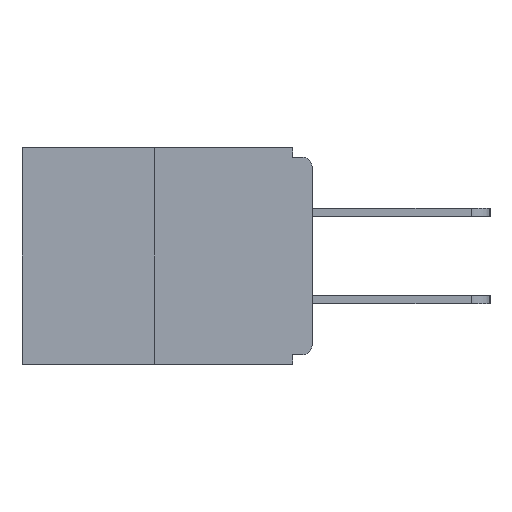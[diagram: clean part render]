
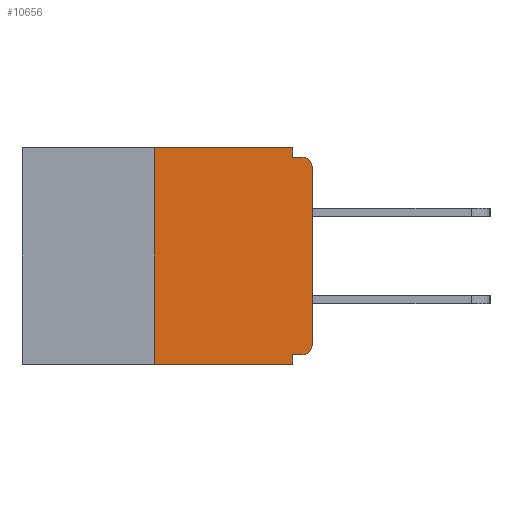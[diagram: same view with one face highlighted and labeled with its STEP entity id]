
A CAD part, left-side view. The second image highlights one B-rep face of the part: STEP entity #10656.
In plain terms, the highlighted planar face has unit normal (-1, 0, 0).
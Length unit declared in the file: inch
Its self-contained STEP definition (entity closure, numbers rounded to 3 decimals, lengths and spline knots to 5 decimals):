
#269 = VERTEX_POINT ( 'NONE', #14708 ) ;
#321 = LINE ( 'NONE', #11312, #3294 ) ;
#499 = VECTOR ( 'NONE', #761, 39.37008 ) ;
#652 = LINE ( 'NONE', #10535, #11108 ) ;
#732 = DIRECTION ( 'NONE',  ( 0., -1., 0. ) ) ;
#761 = DIRECTION ( 'NONE',  ( 0., 0., -1. ) ) ;
#832 = EDGE_CURVE ( 'NONE', #15999, #13995, #10374, .T. ) ;
#1209 = PLANE ( 'NONE',  #2395 ) ;
#1759 = VECTOR ( 'NONE', #14114, 39.37008 ) ;
#1936 = CARTESIAN_POINT ( 'NONE',  ( 0., 0., -0.015 ) ) ;
#2369 = EDGE_CURVE ( 'NONE', #269, #11917, #4774, .T. ) ;
#2395 = AXIS2_PLACEMENT_3D ( 'NONE', #10251, #11724, #10122 ) ;
#2478 = ORIENTED_EDGE ( 'NONE', *, *, #14129, .T. ) ;
#3040 = DIRECTION ( 'NONE',  ( -1., 0., 0. ) ) ;
#3227 = EDGE_LOOP ( 'NONE', ( #15905, #7117, #5791, #7458, #13691, #15611, #5646, #2478, #8967, #14660 ) ) ;
#3228 = AXIS2_PLACEMENT_3D ( 'NONE', #17382, #3040, #4282 ) ;
#3294 = VECTOR ( 'NONE', #17302, 39.37008 ) ;
#3340 = DIRECTION ( 'NONE',  ( 0., 0., 1. ) ) ;
#3433 = LINE ( 'NONE', #5644, #18622 ) ;
#4282 = DIRECTION ( 'NONE',  ( 0., 0., -1. ) ) ;
#4419 = VERTEX_POINT ( 'NONE', #15885 ) ;
#4670 = VECTOR ( 'NONE', #732, 39.37008 ) ;
#4696 = LINE ( 'NONE', #17206, #7650 ) ;
#4774 = LINE ( 'NONE', #10474, #15256 ) ;
#4870 = DIRECTION ( 'NONE',  ( 0., 0., -1. ) ) ;
#5045 = CARTESIAN_POINT ( 'NONE',  ( 0., 0.031, 0. ) ) ;
#5542 = CARTESIAN_POINT ( 'NONE',  ( 0., 0.031, 0. ) ) ;
#5644 = CARTESIAN_POINT ( 'NONE',  ( 0., 0.46, 0. ) ) ;
#5646 = ORIENTED_EDGE ( 'NONE', *, *, #15625, .T. ) ;
#5791 = ORIENTED_EDGE ( 'NONE', *, *, #15986, .T. ) ;
#6509 = LINE ( 'NONE', #12842, #1759 ) ;
#7117 = ORIENTED_EDGE ( 'NONE', *, *, #12773, .F. ) ;
#7458 = ORIENTED_EDGE ( 'NONE', *, *, #2369, .F. ) ;
#7491 = CIRCLE ( 'NONE', #3228, 0.015 ) ;
#7543 = DIRECTION ( 'NONE',  ( -1., 0., 0. ) ) ;
#7650 = VECTOR ( 'NONE', #12997, 39.37008 ) ;
#8511 = CARTESIAN_POINT ( 'NONE',  ( 0., 0.031, -0.015 ) ) ;
#8608 = VERTEX_POINT ( 'NONE', #10536 ) ;
#8967 = ORIENTED_EDGE ( 'NONE', *, *, #832, .F. ) ;
#9833 = EDGE_CURVE ( 'NONE', #15974, #269, #321, .T. ) ;
#10122 = DIRECTION ( 'NONE',  ( 0., 0., -1. ) ) ;
#10251 = CARTESIAN_POINT ( 'NONE',  ( 0., 0.46, 0. ) ) ;
#10374 = LINE ( 'NONE', #1936, #4670 ) ;
#10377 = CARTESIAN_POINT ( 'NONE',  ( 0., 0.015, -0.015 ) ) ;
#10474 = CARTESIAN_POINT ( 'NONE',  ( 0., 0.031, -0.343 ) ) ;
#10514 = CIRCLE ( 'NONE', #13297, 0.015 ) ;
#10535 = CARTESIAN_POINT ( 'NONE',  ( 0., 0.25, 0. ) ) ;
#10536 = CARTESIAN_POINT ( 'NONE',  ( 0., 0.25, -0.343 ) ) ;
#10656 = ADVANCED_FACE ( 'NONE', ( #10712 ), #1209, .F. ) ;
#10712 = FACE_OUTER_BOUND ( 'NONE', #3227, .T. ) ;
#10724 = CARTESIAN_POINT ( 'NONE',  ( 0., 0.015, -0.313 ) ) ;
#10970 = EDGE_CURVE ( 'NONE', #12462, #15999, #11608, .T. ) ;
#11108 = VECTOR ( 'NONE', #3340, 39.37008 ) ;
#11312 = CARTESIAN_POINT ( 'NONE',  ( 0., 0., -0.328 ) ) ;
#11608 = LINE ( 'NONE', #5045, #499 ) ;
#11687 = CARTESIAN_POINT ( 'NONE',  ( 0., 0.25, 0. ) ) ;
#11724 = DIRECTION ( 'NONE',  ( 1., 0., 0. ) ) ;
#11917 = VERTEX_POINT ( 'NONE', #18630 ) ;
#12240 = CARTESIAN_POINT ( 'NONE',  ( 0., 0.015, -0.328 ) ) ;
#12462 = VERTEX_POINT ( 'NONE', #5542 ) ;
#12553 = VERTEX_POINT ( 'NONE', #11687 ) ;
#12773 = EDGE_CURVE ( 'NONE', #8608, #12553, #652, .T. ) ;
#12842 = CARTESIAN_POINT ( 'NONE',  ( 0., 0.46, -0.343 ) ) ;
#12997 = DIRECTION ( 'NONE',  ( 0., 0., 1. ) ) ;
#13297 = AXIS2_PLACEMENT_3D ( 'NONE', #10724, #7543, #4870 ) ;
#13691 = ORIENTED_EDGE ( 'NONE', *, *, #9833, .F. ) ;
#13995 = VERTEX_POINT ( 'NONE', #10377 ) ;
#14114 = DIRECTION ( 'NONE',  ( 0., -1., 0. ) ) ;
#14129 = EDGE_CURVE ( 'NONE', #18629, #13995, #7491, .T. ) ;
#14409 = DIRECTION ( 'NONE',  ( 0., -1., 0. ) ) ;
#14459 = EDGE_CURVE ( 'NONE', #12553, #12462, #3433, .T. ) ;
#14660 = ORIENTED_EDGE ( 'NONE', *, *, #10970, .F. ) ;
#14708 = CARTESIAN_POINT ( 'NONE',  ( 0., 0.031, -0.328 ) ) ;
#15256 = VECTOR ( 'NONE', #16416, 39.37008 ) ;
#15611 = ORIENTED_EDGE ( 'NONE', *, *, #17369, .T. ) ;
#15625 = EDGE_CURVE ( 'NONE', #4419, #18629, #4696, .T. ) ;
#15885 = CARTESIAN_POINT ( 'NONE',  ( 0., 0., -0.313 ) ) ;
#15905 = ORIENTED_EDGE ( 'NONE', *, *, #14459, .F. ) ;
#15974 = VERTEX_POINT ( 'NONE', #12240 ) ;
#15986 = EDGE_CURVE ( 'NONE', #8608, #11917, #6509, .T. ) ;
#15999 = VERTEX_POINT ( 'NONE', #8511 ) ;
#16416 = DIRECTION ( 'NONE',  ( 0., 0., -1. ) ) ;
#17206 = CARTESIAN_POINT ( 'NONE',  ( 0., 0., 0. ) ) ;
#17302 = DIRECTION ( 'NONE',  ( 0., 1., 0. ) ) ;
#17369 = EDGE_CURVE ( 'NONE', #15974, #4419, #10514, .T. ) ;
#17382 = CARTESIAN_POINT ( 'NONE',  ( 0., 0.015, -0.03 ) ) ;
#18029 = CARTESIAN_POINT ( 'NONE',  ( 0., 0., -0.03 ) ) ;
#18622 = VECTOR ( 'NONE', #14409, 39.37008 ) ;
#18629 = VERTEX_POINT ( 'NONE', #18029 ) ;
#18630 = CARTESIAN_POINT ( 'NONE',  ( 0., 0.031, -0.343 ) ) ;
